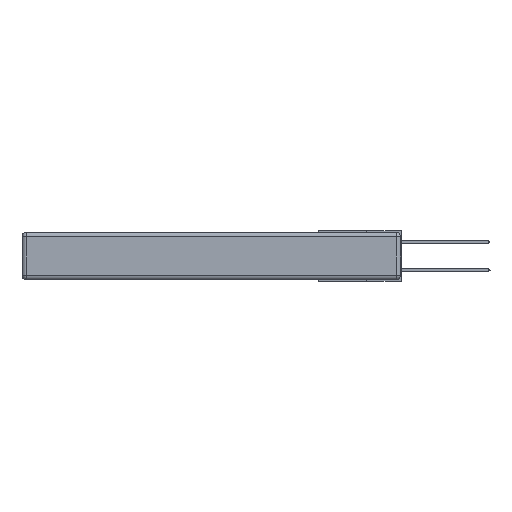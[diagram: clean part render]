
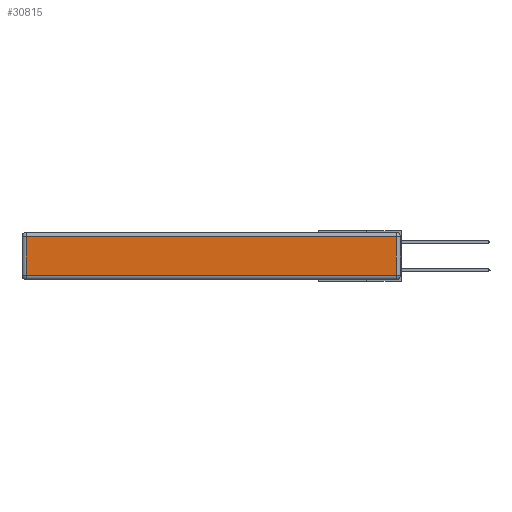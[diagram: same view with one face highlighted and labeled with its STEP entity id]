
A CAD part, left-side view. The second image highlights one B-rep face of the part: STEP entity #30815.
In plain terms, the highlighted planar face has unit normal (-1, 0, 0).
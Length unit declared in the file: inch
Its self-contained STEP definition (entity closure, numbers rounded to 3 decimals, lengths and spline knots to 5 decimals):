
#252 = CARTESIAN_POINT ( 'NONE',  ( 0., 0.03, -0.343 ) ) ;
#1165 = LINE ( 'NONE', #252, #25756 ) ;
#3677 = DIRECTION ( 'NONE',  ( 0., 1., 0. ) ) ;
#4119 = DIRECTION ( 'NONE',  ( -1., 0., 0. ) ) ;
#4315 = VECTOR ( 'NONE', #3677, 39.37008 ) ;
#6305 = PLANE ( 'NONE',  #30423 ) ;
#6419 = CARTESIAN_POINT ( 'NONE',  ( 0., 0.03, -0.313 ) ) ;
#7492 = ORIENTED_EDGE ( 'NONE', *, *, #27810, .T. ) ;
#7641 = FACE_OUTER_BOUND ( 'NONE', #24428, .T. ) ;
#7896 = DIRECTION ( 'NONE',  ( 0., -1., 0. ) ) ;
#8539 = VERTEX_POINT ( 'NONE', #23678 ) ;
#10447 = CARTESIAN_POINT ( 'NONE',  ( 0., 2.72, -0.313 ) ) ;
#12897 = LINE ( 'NONE', #12931, #4315 ) ;
#12931 = CARTESIAN_POINT ( 'NONE',  ( 0., 2.75, -0.03 ) ) ;
#13417 = LINE ( 'NONE', #21041, #24940 ) ;
#14246 = ORIENTED_EDGE ( 'NONE', *, *, #17401, .T. ) ;
#14308 = CARTESIAN_POINT ( 'NONE',  ( 0., 2.72, -0.03 ) ) ;
#14669 = DIRECTION ( 'NONE',  ( 0., 0., 1. ) ) ;
#15113 = CARTESIAN_POINT ( 'NONE',  ( 0., 0., -0.313 ) ) ;
#15658 = LINE ( 'NONE', #15113, #27522 ) ;
#16284 = VERTEX_POINT ( 'NONE', #6419 ) ;
#17158 = VERTEX_POINT ( 'NONE', #14308 ) ;
#17401 = EDGE_CURVE ( 'NONE', #8539, #17158, #12897, .T. ) ;
#18606 = ORIENTED_EDGE ( 'NONE', *, *, #28085, .T. ) ;
#20507 = CARTESIAN_POINT ( 'NONE',  ( 0., 0., -0.343 ) ) ;
#21041 = CARTESIAN_POINT ( 'NONE',  ( 0., 2.72, -0.343 ) ) ;
#22107 = ORIENTED_EDGE ( 'NONE', *, *, #25487, .T. ) ;
#22994 = DIRECTION ( 'NONE',  ( 0., 0., 1. ) ) ;
#23402 = DIRECTION ( 'NONE',  ( 0., 0., -1. ) ) ;
#23678 = CARTESIAN_POINT ( 'NONE',  ( 0., 0.03, -0.03 ) ) ;
#24428 = EDGE_LOOP ( 'NONE', ( #7492, #22107, #14246, #18606 ) ) ;
#24940 = VECTOR ( 'NONE', #23402, 39.37008 ) ;
#25487 = EDGE_CURVE ( 'NONE', #16284, #8539, #1165, .T. ) ;
#25756 = VECTOR ( 'NONE', #14669, 39.37008 ) ;
#27522 = VECTOR ( 'NONE', #7896, 39.37008 ) ;
#27810 = EDGE_CURVE ( 'NONE', #28486, #16284, #15658, .T. ) ;
#28085 = EDGE_CURVE ( 'NONE', #17158, #28486, #13417, .T. ) ;
#28486 = VERTEX_POINT ( 'NONE', #10447 ) ;
#30423 = AXIS2_PLACEMENT_3D ( 'NONE', #20507, #4119, #22994 ) ;
#30815 = ADVANCED_FACE ( 'NONE', ( #7641 ), #6305, .T. ) ;
